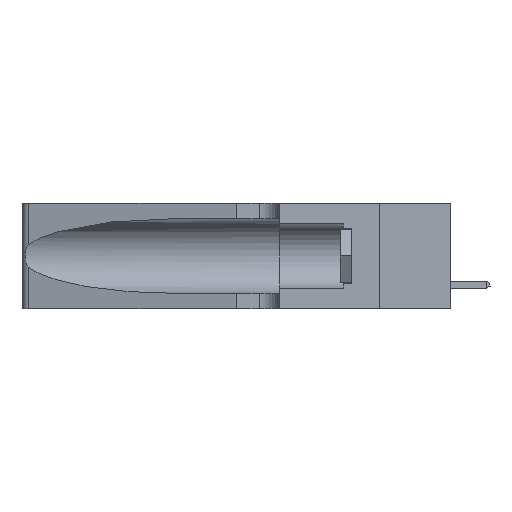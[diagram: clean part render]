
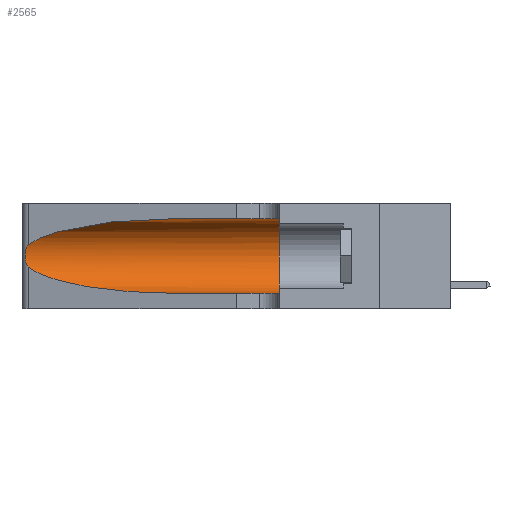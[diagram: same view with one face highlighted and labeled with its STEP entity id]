
A CAD part, left-side view. The second image highlights one B-rep face of the part: STEP entity #2565.
In plain terms, the highlighted cylindrical face has radius 3.308 mm (diameter 6.617 mm), a partial arc.
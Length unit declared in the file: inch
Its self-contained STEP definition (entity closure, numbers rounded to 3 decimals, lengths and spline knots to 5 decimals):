
#973 = CARTESIAN_POINT ( 'NONE',  ( 0.26018, 1.23835, 0.19895 ) ) ;
#1149 = CARTESIAN_POINT ( 'NONE',  ( 0.25856, 1.23593, 0.16098 ) ) ;
#1387 = CARTESIAN_POINT ( 'NONE',  ( 0.1305, 0.72297, 0.31525 ) ) ;
#1633 = EDGE_CURVE ( 'NONE', #9611, #47791, #42651, .T. ) ;
#1937 = CIRCLE ( 'NONE', #16670, 0.13025 ) ;
#2453 = VERTEX_POINT ( 'NONE', #33635 ) ;
#2565 = ADVANCED_FACE ( 'NONE', ( #47959 ), #16448, .F. ) ;
#3325 = CARTESIAN_POINT ( 'NONE',  ( 0.1305, 0.72297, 0.05475 ) ) ;
#4314 = CARTESIAN_POINT ( 'NONE',  ( 0.2373, 1.15595, 0.28018 ) ) ;
#5189 = CARTESIAN_POINT ( 'NONE',  ( 0.25555, 1.22993, 0.14849 ) ) ;
#7281 = CARTESIAN_POINT ( 'NONE',  ( 0.25487, 1.22718, 0.14631 ) ) ;
#7566 = DIRECTION ( 'NONE',  ( 0., -1., 0. ) ) ;
#7702 = EDGE_LOOP ( 'NONE', ( #15113, #15174, #26287, #38962, #19991, #20271 ) ) ;
#9080 = CARTESIAN_POINT ( 'NONE',  ( 0.25487, 1.22718, 0.14631 ) ) ;
#9413 = CARTESIAN_POINT ( 'NONE',  ( 0.1305, 0.35, 0.05475 ) ) ;
#9611 = VERTEX_POINT ( 'NONE', #3325 ) ;
#9804 = VECTOR ( 'NONE', #7566, 39.37008 ) ;
#10158 = CARTESIAN_POINT ( 'NONE',  ( 0.2373, 1.15595, 0.08982 ) ) ;
#13214 = CARTESIAN_POINT ( 'NONE',  ( 0.26075, 1.23896, 0.178 ) ) ;
#14738 = DIRECTION ( 'NONE',  ( 0., -1., 0. ) ) ;
#15113 = ORIENTED_EDGE ( 'NONE', *, *, #19733, .T. ) ;
#15174 = ORIENTED_EDGE ( 'NONE', *, *, #36226, .T. ) ;
#15933 = CARTESIAN_POINT ( 'NONE',  ( 0.1305, 1.61858, 0.31525 ) ) ;
#16380 = DIRECTION ( 'NONE',  ( 0., 1., 0. ) ) ;
#16448 = CYLINDRICAL_SURFACE ( 'NONE', #28114, 0.13025 ) ;
#16591 = DIRECTION ( 'NONE',  ( 0., -1., 0. ) ) ;
#16670 = AXIS2_PLACEMENT_3D ( 'NONE', #25035, #16380, #32291 ) ;
#17626 = CARTESIAN_POINT ( 'NONE',  ( 0.25787, 1.23484, 0.2124 ) ) ;
#17821 = CARTESIAN_POINT ( 'NONE',  ( 0.1305, 0.72297, 0.05475 ) ) ;
#18508 = CARTESIAN_POINT ( 'NONE',  ( 0.18966, 0.96281, 0.05475 ) ) ;
#18944 = EDGE_CURVE ( 'NONE', #35460, #2453, #49580, .T. ) ;
#19278 = VECTOR ( 'NONE', #16591, 39.37008 ) ;
#19733 = EDGE_CURVE ( 'NONE', #35460, #41112, #50542, .T. ) ;
#19991 = ORIENTED_EDGE ( 'NONE', *, *, #45768, .F. ) ;
#20271 = ORIENTED_EDGE ( 'NONE', *, *, #18944, .F. ) ;
#20285 = CARTESIAN_POINT ( 'NONE',  ( 0.1305, 0.72297, 0.31525 ) ) ;
#21350 = CARTESIAN_POINT ( 'NONE',  ( 0.25854, 1.2359, 0.20912 ) ) ;
#21826 = CARTESIAN_POINT ( 'NONE',  ( 0.1305, 1.61858, 0.185 ) ) ;
#24527 = CARTESIAN_POINT ( 'NONE',  ( 0.1305, 1.61858, 0.05475 ) ) ;
#25035 = CARTESIAN_POINT ( 'NONE',  ( 0.1305, 0.35, 0.185 ) ) ;
#25406 = CARTESIAN_POINT ( 'NONE',  ( 0.25487, 1.22718, 0.22369 ) ) ;
#26287 = ORIENTED_EDGE ( 'NONE', *, *, #44687, .T. ) ;
#27111 = DIRECTION ( 'NONE',  ( 0., 0., -1. ) ) ;
#27915 = CARTESIAN_POINT ( 'NONE',  ( 0.25487, 1.22718, 0.22369 ) ) ;
#28114 = AXIS2_PLACEMENT_3D ( 'NONE', #21826, #14738, #27111 ) ;
#29475 = CARTESIAN_POINT ( 'NONE',  ( 0.25639, 1.23186, 0.15144 ) ) ;
#30363 = CARTESIAN_POINT ( 'NONE',  ( 0.25487, 1.22718, 0.14631 ) ) ;
#32291 = DIRECTION ( 'NONE',  ( 0., 0., 1. ) ) ;
#32482 = CARTESIAN_POINT ( 'NONE',  ( 0.18966, 0.96281, 0.31525 ) ) ;
#33356 = CARTESIAN_POINT ( 'NONE',  ( 0.25789, 1.23486, 0.15765 ) ) ;
#33635 = CARTESIAN_POINT ( 'NONE',  ( 0.1305, 0.35, 0.31525 ) ) ;
#33698 = CARTESIAN_POINT ( 'NONE',  ( 0.26075, 1.23896, 0.19203 ) ) ;
#35460 = VERTEX_POINT ( 'NONE', #1387 ) ;
#36226 = EDGE_CURVE ( 'NONE', #41112, #43028, #47629, .T. ) ;
#37230 = CARTESIAN_POINT ( 'NONE',  ( 0.26017, 1.23833, 0.17102 ) ) ;
#38962 = ORIENTED_EDGE ( 'NONE', *, *, #1633, .T. ) ;
#41112 = VERTEX_POINT ( 'NONE', #45575 ) ;
#41815 = CARTESIAN_POINT ( 'NONE',  ( 0.25555, 1.22994, 0.2215 ) ) ;
#42651 = LINE ( 'NONE', #24527, #19278 ) ;
#43028 = VERTEX_POINT ( 'NONE', #7281 ) ;
#44440 =( BOUNDED_CURVE ( )  B_SPLINE_CURVE ( 3, ( #30363, #10158, #18508, #17821 ),
 .UNSPECIFIED., .F., .F. ) 
 B_SPLINE_CURVE_WITH_KNOTS ( ( 4, 4 ),
 ( 3.44316, 4.71239 ),
 .UNSPECIFIED. ) 
 CURVE ( )  GEOMETRIC_REPRESENTATION_ITEM ( )  RATIONAL_B_SPLINE_CURVE ( ( 1., 0.87, 0.87, 1. ) ) 
 REPRESENTATION_ITEM ( '' )  );
#44687 = EDGE_CURVE ( 'NONE', #43028, #9611, #44440, .T. ) ;
#45575 = CARTESIAN_POINT ( 'NONE',  ( 0.25487, 1.22718, 0.22369 ) ) ;
#45768 = EDGE_CURVE ( 'NONE', #2453, #47791, #1937, .T. ) ;
#45845 = CARTESIAN_POINT ( 'NONE',  ( 0.25639, 1.23184, 0.21858 ) ) ;
#47629 = B_SPLINE_CURVE_WITH_KNOTS ( 'NONE', 3,
 ( #25406, #41815, #45845, #17626, #21350, #973, #33698, #13214, #37230, #1149, #33356, #29475, #5189, #9080 ),
 .UNSPECIFIED., .F., .F.,
 ( 4, 2, 2, 2, 2, 2, 4 ),
 ( 0., 0.00027, 0.00053, 0.00107, 0.0016, 0.00187, 0.00214 ),
 .UNSPECIFIED. ) ;
#47791 = VERTEX_POINT ( 'NONE', #9413 ) ;
#47959 = FACE_OUTER_BOUND ( 'NONE', #7702, .T. ) ;
#49580 = LINE ( 'NONE', #15933, #9804 ) ;
#50542 =( BOUNDED_CURVE ( )  B_SPLINE_CURVE ( 3, ( #20285, #32482, #4314, #27915 ),
 .UNSPECIFIED., .F., .T. ) 
 B_SPLINE_CURVE_WITH_KNOTS ( ( 4, 4 ),
 ( 1.5708, 2.84003 ),
 .UNSPECIFIED. ) 
 CURVE ( )  GEOMETRIC_REPRESENTATION_ITEM ( )  RATIONAL_B_SPLINE_CURVE ( ( 1., 0.87, 0.87, 1. ) ) 
 REPRESENTATION_ITEM ( '' )  );
